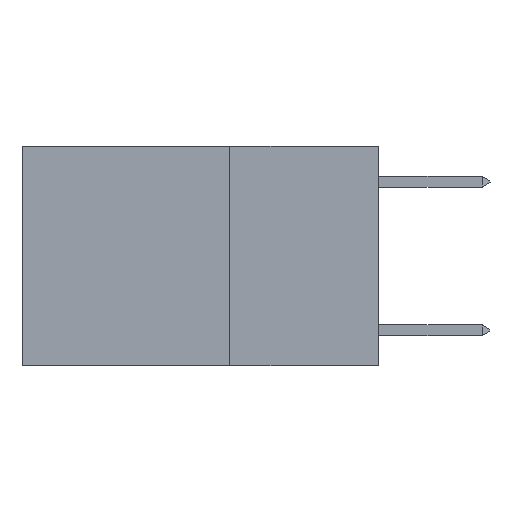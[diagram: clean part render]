
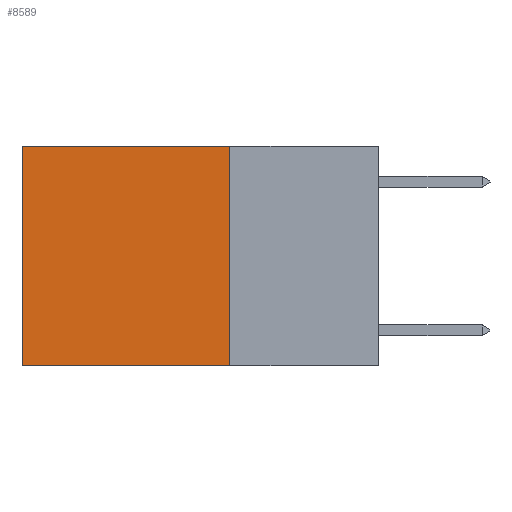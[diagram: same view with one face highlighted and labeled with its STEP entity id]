
A CAD part, left-side view. The second image highlights one B-rep face of the part: STEP entity #8589.
In plain terms, the highlighted planar face has unit normal (-1, 0, 0).
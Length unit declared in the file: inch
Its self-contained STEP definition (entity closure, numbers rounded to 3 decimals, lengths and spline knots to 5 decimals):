
#383 = LINE ( 'NONE', #561, #3916 ) ;
#561 = CARTESIAN_POINT ( 'NONE',  ( 0.2625, 0.6, 0. ) ) ;
#659 = ORIENTED_EDGE ( 'NONE', *, *, #7950, .F. ) ;
#706 = PLANE ( 'NONE',  #1026 ) ;
#904 = VECTOR ( 'NONE', #6543, 39.37008 ) ;
#1026 = AXIS2_PLACEMENT_3D ( 'NONE', #8395, #6786, #7748 ) ;
#1288 = ORIENTED_EDGE ( 'NONE', *, *, #6747, .T. ) ;
#2383 = CARTESIAN_POINT ( 'NONE',  ( 0.2625, 0.25, 0. ) ) ;
#3303 = CARTESIAN_POINT ( 'NONE',  ( 0.2625, 0.25, 0. ) ) ;
#3610 = DIRECTION ( 'NONE',  ( 0., 0., -1. ) ) ;
#3735 = EDGE_LOOP ( 'NONE', ( #4010, #3768, #659, #1288 ) ) ;
#3768 = ORIENTED_EDGE ( 'NONE', *, *, #6012, .F. ) ;
#3916 = VECTOR ( 'NONE', #3610, 39.37008 ) ;
#4010 = ORIENTED_EDGE ( 'NONE', *, *, #4790, .T. ) ;
#4031 = VERTEX_POINT ( 'NONE', #8614 ) ;
#4083 = CARTESIAN_POINT ( 'NONE',  ( 0.2625, 0.6, -0.37 ) ) ;
#4216 = VERTEX_POINT ( 'NONE', #4083 ) ;
#4239 = CARTESIAN_POINT ( 'NONE',  ( 0.2625, 0.6, 0. ) ) ;
#4424 = VECTOR ( 'NONE', #4859, 39.37008 ) ;
#4454 = LINE ( 'NONE', #4498, #9182 ) ;
#4498 = CARTESIAN_POINT ( 'NONE',  ( 0.2625, 0.25, 0. ) ) ;
#4510 = FACE_OUTER_BOUND ( 'NONE', #3735, .T. ) ;
#4790 = EDGE_CURVE ( 'NONE', #8741, #4216, #383, .T. ) ;
#4859 = DIRECTION ( 'NONE',  ( 0., 1., 0. ) ) ;
#5566 = LINE ( 'NONE', #3303, #4424 ) ;
#6012 = EDGE_CURVE ( 'NONE', #4031, #4216, #9723, .T. ) ;
#6054 = DIRECTION ( 'NONE',  ( 0., 0., -1. ) ) ;
#6543 = DIRECTION ( 'NONE',  ( 0., 1., 0. ) ) ;
#6747 = EDGE_CURVE ( 'NONE', #7545, #8741, #5566, .T. ) ;
#6786 = DIRECTION ( 'NONE',  ( 1., 0., 0. ) ) ;
#7545 = VERTEX_POINT ( 'NONE', #2383 ) ;
#7748 = DIRECTION ( 'NONE',  ( 0., 0., -1. ) ) ;
#7950 = EDGE_CURVE ( 'NONE', #7545, #4031, #4454, .T. ) ;
#8395 = CARTESIAN_POINT ( 'NONE',  ( 0.2625, 0.25, 0. ) ) ;
#8589 = ADVANCED_FACE ( 'NONE', ( #4510 ), #706, .F. ) ;
#8614 = CARTESIAN_POINT ( 'NONE',  ( 0.2625, 0.25, -0.37 ) ) ;
#8741 = VERTEX_POINT ( 'NONE', #4239 ) ;
#8752 = CARTESIAN_POINT ( 'NONE',  ( 0.2625, 0.25, -0.37 ) ) ;
#9182 = VECTOR ( 'NONE', #6054, 39.37008 ) ;
#9723 = LINE ( 'NONE', #8752, #904 ) ;
